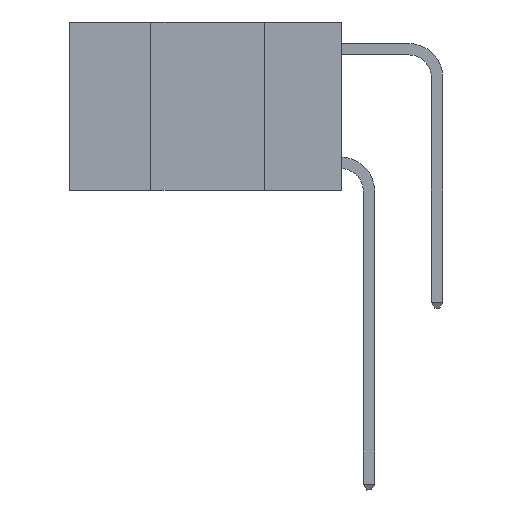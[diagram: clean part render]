
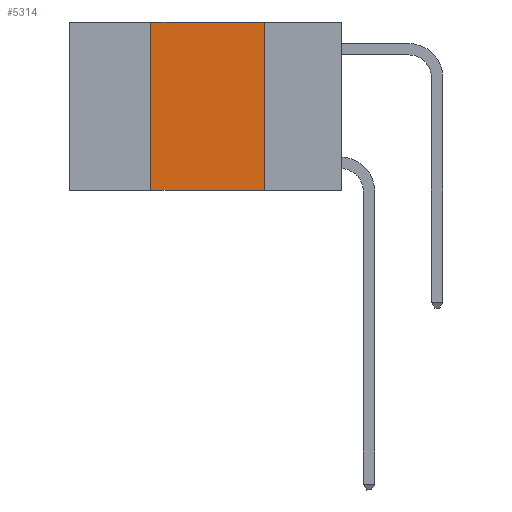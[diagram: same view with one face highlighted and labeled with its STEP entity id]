
A CAD part, left-side view. The second image highlights one B-rep face of the part: STEP entity #5314.
In plain terms, the highlighted planar face has unit normal (-1, 0, 0).
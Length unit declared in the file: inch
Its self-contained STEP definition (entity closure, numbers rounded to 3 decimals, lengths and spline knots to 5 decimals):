
#365 = ORIENTED_EDGE ( 'NONE', *, *, #10922, .F. ) ;
#937 = ORIENTED_EDGE ( 'NONE', *, *, #10386, .F. ) ;
#1170 = VECTOR ( 'NONE', #19995, 39.37008 ) ;
#1500 = EDGE_LOOP ( 'NONE', ( #365, #5085, #937, #8805 ) ) ;
#2009 = CARTESIAN_POINT ( 'NONE',  ( 0., 0.6, 0. ) ) ;
#3479 = LINE ( 'NONE', #5639, #15644 ) ;
#3504 = CARTESIAN_POINT ( 'NONE',  ( 0., 0.17, -0.37 ) ) ;
#3805 = DIRECTION ( 'NONE',  ( 0., 0., -1. ) ) ;
#4162 = CARTESIAN_POINT ( 'NONE',  ( 0., 0.42, 0. ) ) ;
#5085 = ORIENTED_EDGE ( 'NONE', *, *, #6228, .F. ) ;
#5314 = ADVANCED_FACE ( 'NONE', ( #5410 ), #8304, .F. ) ;
#5410 = FACE_OUTER_BOUND ( 'NONE', #1500, .T. ) ;
#5639 = CARTESIAN_POINT ( 'NONE',  ( 0., 0.6, -0.37 ) ) ;
#6228 = EDGE_CURVE ( 'NONE', #14124, #6665, #13810, .T. ) ;
#6665 = VERTEX_POINT ( 'NONE', #12878 ) ;
#8304 = PLANE ( 'NONE',  #18459 ) ;
#8536 = VERTEX_POINT ( 'NONE', #3504 ) ;
#8777 = EDGE_CURVE ( 'NONE', #11745, #8536, #3479, .T. ) ;
#8805 = ORIENTED_EDGE ( 'NONE', *, *, #8777, .T. ) ;
#9915 = DIRECTION ( 'NONE',  ( 0., 0., -1. ) ) ;
#10369 = DIRECTION ( 'NONE',  ( 0., 0., 1. ) ) ;
#10386 = EDGE_CURVE ( 'NONE', #11745, #14124, #16600, .T. ) ;
#10922 = EDGE_CURVE ( 'NONE', #6665, #8536, #19304, .T. ) ;
#11745 = VERTEX_POINT ( 'NONE', #15226 ) ;
#12378 = VECTOR ( 'NONE', #10369, 39.37008 ) ;
#12550 = CARTESIAN_POINT ( 'NONE',  ( 0., 0.42, 0. ) ) ;
#12878 = CARTESIAN_POINT ( 'NONE',  ( 0., 0.17, 0. ) ) ;
#13617 = DIRECTION ( 'NONE',  ( 0., -1., 0. ) ) ;
#13810 = LINE ( 'NONE', #15157, #1170 ) ;
#14124 = VERTEX_POINT ( 'NONE', #12550 ) ;
#15092 = VECTOR ( 'NONE', #3805, 39.37008 ) ;
#15157 = CARTESIAN_POINT ( 'NONE',  ( 0., 0.6, 0. ) ) ;
#15226 = CARTESIAN_POINT ( 'NONE',  ( 0., 0.42, -0.37 ) ) ;
#15644 = VECTOR ( 'NONE', #13617, 39.37008 ) ;
#16474 = CARTESIAN_POINT ( 'NONE',  ( 0., 0.17, 0. ) ) ;
#16600 = LINE ( 'NONE', #4162, #12378 ) ;
#18459 = AXIS2_PLACEMENT_3D ( 'NONE', #2009, #19476, #9915 ) ;
#19304 = LINE ( 'NONE', #16474, #15092 ) ;
#19476 = DIRECTION ( 'NONE',  ( 1., 0., 0. ) ) ;
#19995 = DIRECTION ( 'NONE',  ( 0., -1., 0. ) ) ;
